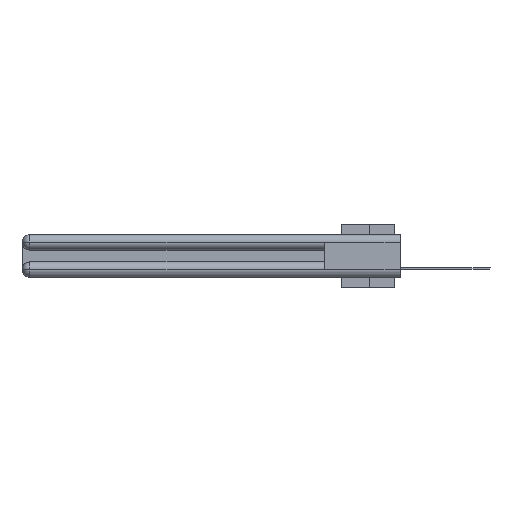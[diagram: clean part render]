
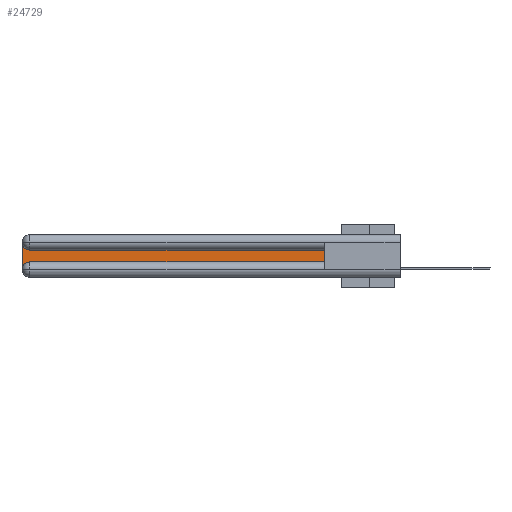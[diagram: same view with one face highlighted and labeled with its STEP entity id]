
A CAD part, left-side view. The second image highlights one B-rep face of the part: STEP entity #24729.
In plain terms, the highlighted planar face has unit normal (-1, 0, 0).
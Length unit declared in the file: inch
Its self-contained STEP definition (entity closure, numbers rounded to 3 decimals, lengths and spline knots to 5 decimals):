
#1070 = DIRECTION ( 'NONE',  ( 1., 0., 0. ) ) ;
#1855 = VECTOR ( 'NONE', #8476, 39.37008 ) ;
#2069 = EDGE_CURVE ( 'NONE', #20271, #25950, #6177, .T. ) ;
#2211 = CARTESIAN_POINT ( 'NONE',  ( 0.075, 2.94, -0.0625 ) ) ;
#2611 = DIRECTION ( 'NONE',  ( 1., 0., 0. ) ) ;
#2717 = ORIENTED_EDGE ( 'NONE', *, *, #2069, .T. ) ;
#2752 = EDGE_CURVE ( 'NONE', #23861, #24570, #16896, .T. ) ;
#4055 = DIRECTION ( 'NONE',  ( 0., 1., 0. ) ) ;
#6177 = CIRCLE ( 'NONE', #8292, 0.06 ) ;
#7094 = CARTESIAN_POINT ( 'NONE',  ( 0.075, 0.6, -0.2175 ) ) ;
#7729 = CARTESIAN_POINT ( 'NONE',  ( 0.075, 2.94, -0.2775 ) ) ;
#8292 = AXIS2_PLACEMENT_3D ( 'NONE', #7729, #2611, #28086 ) ;
#8441 = EDGE_CURVE ( 'NONE', #25950, #31968, #17042, .T. ) ;
#8476 = DIRECTION ( 'NONE',  ( 0., 0., 1. ) ) ;
#8937 = VERTEX_POINT ( 'NONE', #29737 ) ;
#9149 = ORIENTED_EDGE ( 'NONE', *, *, #9673, .T. ) ;
#9673 = EDGE_CURVE ( 'NONE', #8937, #23861, #24573, .T. ) ;
#9913 = DIRECTION ( 'NONE',  ( 0., 0., -1. ) ) ;
#12287 = DIRECTION ( 'NONE',  ( 1., 0., 0. ) ) ;
#12990 = CARTESIAN_POINT ( 'NONE',  ( 0.075, 3., -0.0625 ) ) ;
#13733 = AXIS2_PLACEMENT_3D ( 'NONE', #31717, #1070, #26226 ) ;
#13922 = LINE ( 'NONE', #21062, #1855 ) ;
#13978 = CARTESIAN_POINT ( 'NONE',  ( 0.075, 0.6, -0.1225 ) ) ;
#14046 = DIRECTION ( 'NONE',  ( 0., -1., 0. ) ) ;
#14470 = EDGE_CURVE ( 'NONE', #24570, #20271, #19924, .T. ) ;
#15704 = ORIENTED_EDGE ( 'NONE', *, *, #2752, .T. ) ;
#16139 = FACE_OUTER_BOUND ( 'NONE', #29735, .T. ) ;
#16152 = ORIENTED_EDGE ( 'NONE', *, *, #17546, .T. ) ;
#16896 = CIRCLE ( 'NONE', #30087, 0.06 ) ;
#17042 = LINE ( 'NONE', #7094, #25302 ) ;
#17546 = EDGE_CURVE ( 'NONE', #31968, #8937, #13922, .T. ) ;
#17559 = CARTESIAN_POINT ( 'NONE',  ( 0.075, 3., -0.2175 ) ) ;
#19924 = LINE ( 'NONE', #17559, #28148 ) ;
#20271 = VERTEX_POINT ( 'NONE', #26880 ) ;
#20557 = VECTOR ( 'NONE', #4055, 39.37008 ) ;
#20982 = ORIENTED_EDGE ( 'NONE', *, *, #8441, .T. ) ;
#21062 = CARTESIAN_POINT ( 'NONE',  ( 0.075, 0.6, -0.2175 ) ) ;
#21799 = ORIENTED_EDGE ( 'NONE', *, *, #14470, .T. ) ;
#22290 = CARTESIAN_POINT ( 'NONE',  ( 0.075, 0.6, -0.2175 ) ) ;
#23586 = PLANE ( 'NONE',  #13733 ) ;
#23861 = VERTEX_POINT ( 'NONE', #24880 ) ;
#24556 = DIRECTION ( 'NONE',  ( 0., 0., -1. ) ) ;
#24570 = VERTEX_POINT ( 'NONE', #12990 ) ;
#24573 = LINE ( 'NONE', #13978, #20557 ) ;
#24729 = ADVANCED_FACE ( 'NONE', ( #16139 ), #23586, .F. ) ;
#24880 = CARTESIAN_POINT ( 'NONE',  ( 0.075, 2.94, -0.1225 ) ) ;
#25302 = VECTOR ( 'NONE', #14046, 39.37008 ) ;
#25431 = CARTESIAN_POINT ( 'NONE',  ( 0.075, 2.94, -0.2175 ) ) ;
#25950 = VERTEX_POINT ( 'NONE', #25431 ) ;
#26226 = DIRECTION ( 'NONE',  ( 0., 0., -1. ) ) ;
#26880 = CARTESIAN_POINT ( 'NONE',  ( 0.075, 3., -0.2775 ) ) ;
#28086 = DIRECTION ( 'NONE',  ( 0., 0., -1. ) ) ;
#28148 = VECTOR ( 'NONE', #9913, 39.37008 ) ;
#29735 = EDGE_LOOP ( 'NONE', ( #9149, #15704, #21799, #2717, #20982, #16152 ) ) ;
#29737 = CARTESIAN_POINT ( 'NONE',  ( 0.075, 0.6, -0.1225 ) ) ;
#30087 = AXIS2_PLACEMENT_3D ( 'NONE', #2211, #12287, #24556 ) ;
#31717 = CARTESIAN_POINT ( 'NONE',  ( 0.075, 3., -0.1225 ) ) ;
#31968 = VERTEX_POINT ( 'NONE', #22290 ) ;
